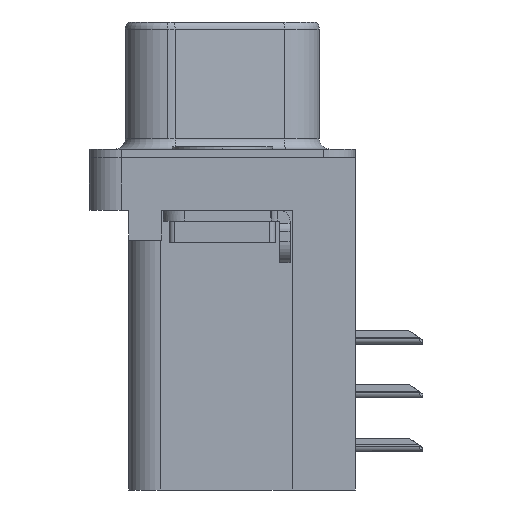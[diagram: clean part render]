
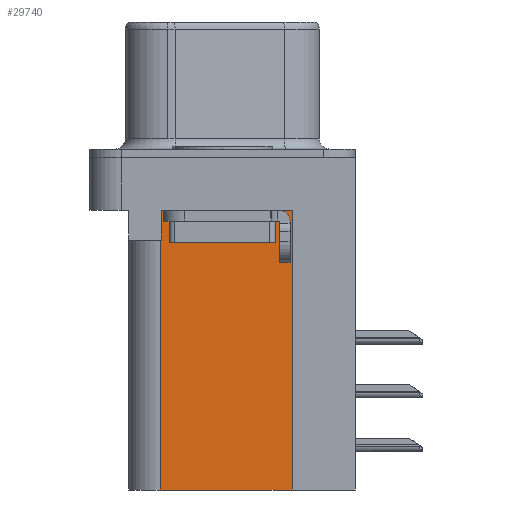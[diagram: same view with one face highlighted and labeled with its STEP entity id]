
A CAD part, left-side view. The second image highlights one B-rep face of the part: STEP entity #29740.
In plain terms, the highlighted planar face has unit normal (-1, 0, 0).
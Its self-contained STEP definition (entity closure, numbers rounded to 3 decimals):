
#1100 = VERTEX_POINT ( 'NONE', #5025 ) ;
#1836 = CARTESIAN_POINT ( 'NONE',  ( 3.79, -3.295, -15.7 ) ) ;
#1988 = VECTOR ( 'NONE', #27374, 1000. ) ;
#2450 = DIRECTION ( 'NONE',  ( 1., 0., 0. ) ) ;
#2972 = DIRECTION ( 'NONE',  ( 0., 1., 0. ) ) ;
#3170 = VERTEX_POINT ( 'NONE', #9458 ) ;
#3424 = ORIENTED_EDGE ( 'NONE', *, *, #6617, .F. ) ;
#4884 = ORIENTED_EDGE ( 'NONE', *, *, #7644, .F. ) ;
#5025 = CARTESIAN_POINT ( 'NONE',  ( 3.79, 2.925, -15.7 ) ) ;
#5273 = LINE ( 'NONE', #14381, #24874 ) ;
#5589 = LINE ( 'NONE', #10720, #30964 ) ;
#5959 = CARTESIAN_POINT ( 'NONE',  ( 3.79, 2.925, -3.9 ) ) ;
#6617 = EDGE_CURVE ( 'NONE', #1100, #26632, #22892, .T. ) ;
#7397 = VECTOR ( 'NONE', #9202, 1000. ) ;
#7581 = ORIENTED_EDGE ( 'NONE', *, *, #19740, .T. ) ;
#7644 = EDGE_CURVE ( 'NONE', #28014, #1100, #5273, .T. ) ;
#7740 = EDGE_CURVE ( 'NONE', #28014, #3170, #22392, .T. ) ;
#8329 = CARTESIAN_POINT ( 'NONE',  ( 3.79, 2.895, -2.5 ) ) ;
#9202 = DIRECTION ( 'NONE',  ( 0., 1., 0. ) ) ;
#9458 = CARTESIAN_POINT ( 'NONE',  ( 3.79, -3.295, -2.5 ) ) ;
#9901 = AXIS2_PLACEMENT_3D ( 'NONE', #30399, #2450, #20382 ) ;
#10585 = CARTESIAN_POINT ( 'NONE',  ( 3.79, 2.895, -3.9 ) ) ;
#10720 = CARTESIAN_POINT ( 'NONE',  ( 3.79, 0., -3.9 ) ) ;
#11766 = FACE_OUTER_BOUND ( 'NONE', #31696, .T. ) ;
#12188 = LINE ( 'NONE', #26992, #31548 ) ;
#12280 = CARTESIAN_POINT ( 'NONE',  ( 3.79, 2.925, -15.7 ) ) ;
#13243 = ORIENTED_EDGE ( 'NONE', *, *, #31741, .T. ) ;
#14300 = DIRECTION ( 'NONE',  ( 0., 0., -1. ) ) ;
#14381 = CARTESIAN_POINT ( 'NONE',  ( 3.79, -3.295, -15.7 ) ) ;
#14909 = DIRECTION ( 'NONE',  ( 0., 0., 1. ) ) ;
#15387 = VECTOR ( 'NONE', #14909, 1000. ) ;
#17871 = VERTEX_POINT ( 'NONE', #10585 ) ;
#19740 = EDGE_CURVE ( 'NONE', #17871, #26632, #5589, .T. ) ;
#20086 = CARTESIAN_POINT ( 'NONE',  ( 3.79, -3.295, -15.7 ) ) ;
#20382 = DIRECTION ( 'NONE',  ( 0., 0., -1. ) ) ;
#21711 = ORIENTED_EDGE ( 'NONE', *, *, #7740, .T. ) ;
#21906 = CARTESIAN_POINT ( 'NONE',  ( 3.79, -3.295, -2.5 ) ) ;
#22392 = LINE ( 'NONE', #1836, #1988 ) ;
#22892 = LINE ( 'NONE', #12280, #15387 ) ;
#24874 = VECTOR ( 'NONE', #29301, 1000. ) ;
#25459 = PLANE ( 'NONE',  #9901 ) ;
#26632 = VERTEX_POINT ( 'NONE', #5959 ) ;
#26992 = CARTESIAN_POINT ( 'NONE',  ( 3.79, 2.895, -3.9 ) ) ;
#27374 = DIRECTION ( 'NONE',  ( 0., 0., 1. ) ) ;
#28014 = VERTEX_POINT ( 'NONE', #20086 ) ;
#28092 = ORIENTED_EDGE ( 'NONE', *, *, #29595, .T. ) ;
#28511 = LINE ( 'NONE', #21906, #7397 ) ;
#29301 = DIRECTION ( 'NONE',  ( 0., 1., 0. ) ) ;
#29595 = EDGE_CURVE ( 'NONE', #3170, #32750, #28511, .T. ) ;
#29740 = ADVANCED_FACE ( 'NONE', ( #11766 ), #25459, .F. ) ;
#30399 = CARTESIAN_POINT ( 'NONE',  ( 3.79, -3.295, -15.7 ) ) ;
#30964 = VECTOR ( 'NONE', #2972, 1000. ) ;
#31548 = VECTOR ( 'NONE', #14300, 1000. ) ;
#31696 = EDGE_LOOP ( 'NONE', ( #28092, #13243, #7581, #3424, #4884, #21711 ) ) ;
#31741 = EDGE_CURVE ( 'NONE', #32750, #17871, #12188, .T. ) ;
#32750 = VERTEX_POINT ( 'NONE', #8329 ) ;
